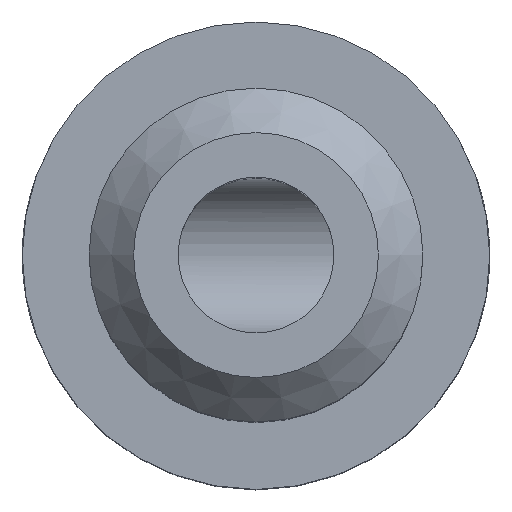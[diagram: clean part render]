
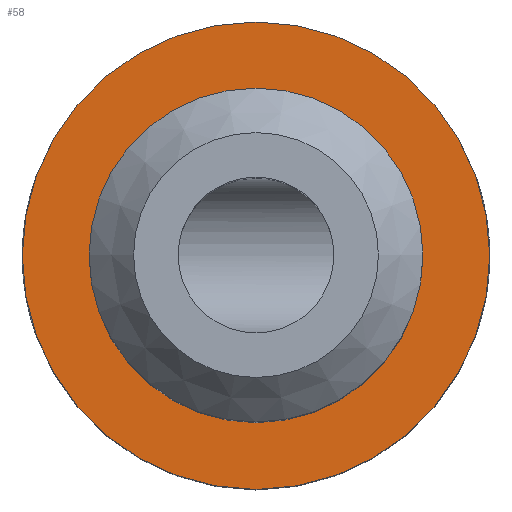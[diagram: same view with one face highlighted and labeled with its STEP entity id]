
A CAD part, top view. The second image highlights one B-rep face of the part: STEP entity #58.
In plain terms, the highlighted planar face has unit normal (0, 0, 1).
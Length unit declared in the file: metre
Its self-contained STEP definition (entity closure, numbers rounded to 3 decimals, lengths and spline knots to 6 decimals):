
#58 = ADVANCED_FACE( '', ( #123, #124 ), #125, .T. );
#123 = FACE_BOUND( '', #180, .T. );
#124 = FACE_OUTER_BOUND( '', #181, .T. );
#125 = PLANE( '', #182 );
#180 = EDGE_LOOP( '', ( #255 ) );
#181 = EDGE_LOOP( '', ( #256 ) );
#182 = AXIS2_PLACEMENT_3D( '', #257, #258, #259 );
#255 = ORIENTED_EDGE( '', *, *, #284, .F. );
#256 = ORIENTED_EDGE( '', *, *, #271, .T. );
#257 = CARTESIAN_POINT( '', ( 0., 0., 0. ) );
#258 = DIRECTION( '', ( 0., 0., 1. ) );
#259 = DIRECTION( '', ( 1., 0., 0. ) );
#271 = EDGE_CURVE( '', #303, #303, #304, .T. );
#284 = EDGE_CURVE( '', #323, #323, #324, .T. );
#303 = VERTEX_POINT( '', #343 );
#304 = CIRCLE( '', #344, 0.00525 );
#323 = VERTEX_POINT( '', #473 );
#324 = CIRCLE( '', #474, 0.00375 );
#343 = CARTESIAN_POINT( '', ( 0.00525, 0., 0. ) );
#344 = AXIS2_PLACEMENT_3D( '', #494, #495, #496 );
#473 = CARTESIAN_POINT( '', ( 0.00375, 0., 0. ) );
#474 = AXIS2_PLACEMENT_3D( '', #509, #510, #511 );
#494 = CARTESIAN_POINT( '', ( 0., 0., 0. ) );
#495 = DIRECTION( '', ( 0., 0., 1. ) );
#496 = DIRECTION( '', ( 1., 0., 0. ) );
#509 = CARTESIAN_POINT( '', ( 0., 0., 0. ) );
#510 = DIRECTION( '', ( 0., 0., 1. ) );
#511 = DIRECTION( '', ( 1., 0., 0. ) );
